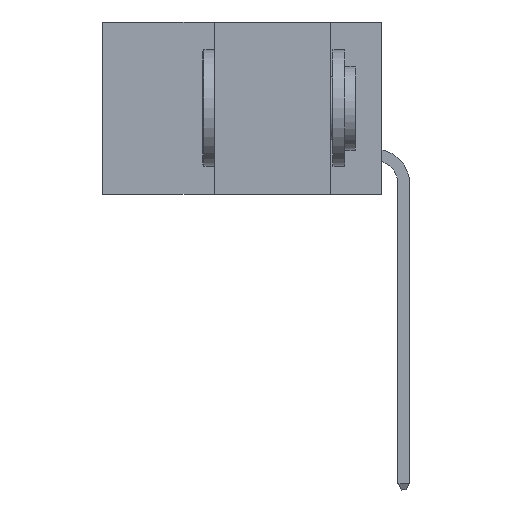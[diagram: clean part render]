
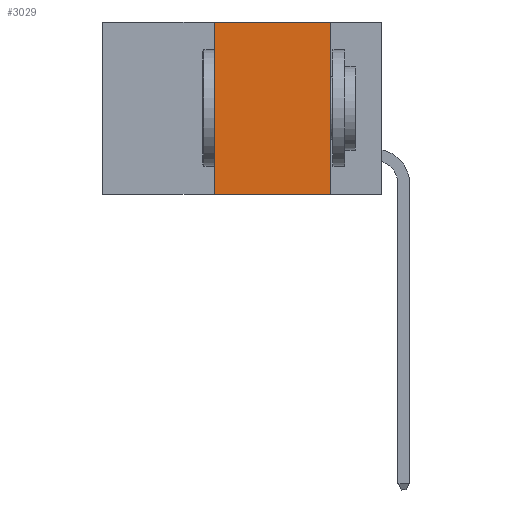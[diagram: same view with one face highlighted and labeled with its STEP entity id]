
A CAD part, left-side view. The second image highlights one B-rep face of the part: STEP entity #3029.
In plain terms, the highlighted planar face has unit normal (-1, 0, 0).
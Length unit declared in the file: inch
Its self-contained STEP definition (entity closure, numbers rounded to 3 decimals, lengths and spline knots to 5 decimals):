
#268 = LINE ( 'NONE', #32680, #20189 ) ;
#400 = CARTESIAN_POINT ( 'NONE',  ( 0., 0.6, 0. ) ) ;
#3029 = ADVANCED_FACE ( 'NONE', ( #22127 ), #10615, .F. ) ;
#3511 = EDGE_CURVE ( 'NONE', #4162, #23990, #28728, .T. ) ;
#4162 = VERTEX_POINT ( 'NONE', #15201 ) ;
#4618 = VERTEX_POINT ( 'NONE', #25066 ) ;
#5223 = CARTESIAN_POINT ( 'NONE',  ( 0., 0.36, 0. ) ) ;
#5564 = DIRECTION ( 'NONE',  ( 0., 0., -1. ) ) ;
#7305 = DIRECTION ( 'NONE',  ( 0., -1., 0. ) ) ;
#7365 = VERTEX_POINT ( 'NONE', #25520 ) ;
#7781 = DIRECTION ( 'NONE',  ( 0., 0., 1. ) ) ;
#7965 = AXIS2_PLACEMENT_3D ( 'NONE', #400, #21184, #5564 ) ;
#8920 = ORIENTED_EDGE ( 'NONE', *, *, #10462, .F. ) ;
#10462 = EDGE_CURVE ( 'NONE', #7365, #23990, #27165, .T. ) ;
#10615 = PLANE ( 'NONE',  #7965 ) ;
#10636 = ORIENTED_EDGE ( 'NONE', *, *, #16475, .F. ) ;
#12203 = ORIENTED_EDGE ( 'NONE', *, *, #3511, .T. ) ;
#13675 = ORIENTED_EDGE ( 'NONE', *, *, #18673, .F. ) ;
#15201 = CARTESIAN_POINT ( 'NONE',  ( 0., 0.36, -0.37 ) ) ;
#16475 = EDGE_CURVE ( 'NONE', #4162, #4618, #28185, .T. ) ;
#18270 = DIRECTION ( 'NONE',  ( 0., 0., -1. ) ) ;
#18673 = EDGE_CURVE ( 'NONE', #4618, #7365, #268, .T. ) ;
#19429 = EDGE_LOOP ( 'NONE', ( #8920, #13675, #10636, #12203 ) ) ;
#20189 = VECTOR ( 'NONE', #30447, 39.37008 ) ;
#20356 = CARTESIAN_POINT ( 'NONE',  ( 0., 0.6, -0.37 ) ) ;
#20702 = VECTOR ( 'NONE', #7781, 39.37008 ) ;
#21184 = DIRECTION ( 'NONE',  ( 1., 0., 0. ) ) ;
#21277 = VECTOR ( 'NONE', #7305, 39.37008 ) ;
#22127 = FACE_OUTER_BOUND ( 'NONE', #19429, .T. ) ;
#23990 = VERTEX_POINT ( 'NONE', #26261 ) ;
#25066 = CARTESIAN_POINT ( 'NONE',  ( 0., 0.36, 0. ) ) ;
#25520 = CARTESIAN_POINT ( 'NONE',  ( 0., 0.11, 0. ) ) ;
#25856 = CARTESIAN_POINT ( 'NONE',  ( 0., 0.11, 0. ) ) ;
#26261 = CARTESIAN_POINT ( 'NONE',  ( 0., 0.11, -0.37 ) ) ;
#27165 = LINE ( 'NONE', #25856, #32891 ) ;
#28185 = LINE ( 'NONE', #5223, #20702 ) ;
#28728 = LINE ( 'NONE', #20356, #21277 ) ;
#30447 = DIRECTION ( 'NONE',  ( 0., -1., 0. ) ) ;
#32680 = CARTESIAN_POINT ( 'NONE',  ( 0., 0.6, 0. ) ) ;
#32891 = VECTOR ( 'NONE', #18270, 39.37008 ) ;
